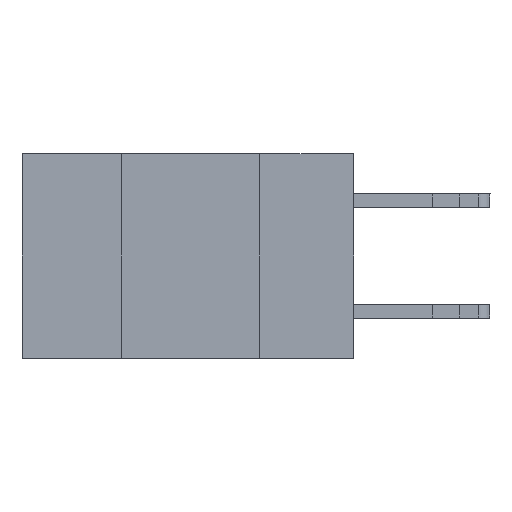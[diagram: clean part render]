
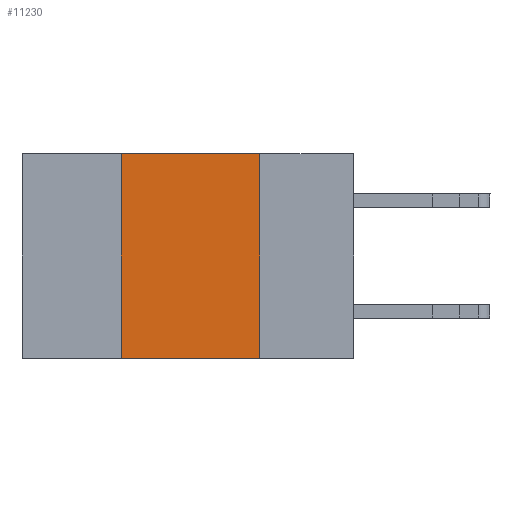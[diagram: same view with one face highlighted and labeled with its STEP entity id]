
A CAD part, left-side view. The second image highlights one B-rep face of the part: STEP entity #11230.
In plain terms, the highlighted planar face has unit normal (-1, 0, 0).
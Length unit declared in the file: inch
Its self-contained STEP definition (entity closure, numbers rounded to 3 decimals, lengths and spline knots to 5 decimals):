
#27 = VECTOR ( 'NONE', #18853, 39.37008 ) ;
#811 = VERTEX_POINT ( 'NONE', #19959 ) ;
#1040 = DIRECTION ( 'NONE',  ( 0., 0., 1. ) ) ;
#1894 = ORIENTED_EDGE ( 'NONE', *, *, #13510, .T. ) ;
#2564 = EDGE_LOOP ( 'NONE', ( #18502, #21080, #18446, #1894 ) ) ;
#2860 = DIRECTION ( 'NONE',  ( 0., -1., 0. ) ) ;
#4408 = LINE ( 'NONE', #16686, #27 ) ;
#8374 = DIRECTION ( 'NONE',  ( 1., 0., 0. ) ) ;
#9602 = AXIS2_PLACEMENT_3D ( 'NONE', #18667, #8374, #18539 ) ;
#10160 = VERTEX_POINT ( 'NONE', #21733 ) ;
#11166 = CARTESIAN_POINT ( 'NONE',  ( 0., 0.42, -0.37 ) ) ;
#11230 = ADVANCED_FACE ( 'NONE', ( #16837 ), #21931, .F. ) ;
#11403 = CARTESIAN_POINT ( 'NONE',  ( 0., 0.6, 0. ) ) ;
#11689 = EDGE_CURVE ( 'NONE', #811, #10160, #14798, .T. ) ;
#12183 = VERTEX_POINT ( 'NONE', #16342 ) ;
#13083 = DIRECTION ( 'NONE',  ( 0., -1., 0. ) ) ;
#13177 = VECTOR ( 'NONE', #1040, 39.37008 ) ;
#13510 = EDGE_CURVE ( 'NONE', #22340, #12183, #16766, .T. ) ;
#14726 = VECTOR ( 'NONE', #2860, 39.37008 ) ;
#14798 = LINE ( 'NONE', #11403, #14726 ) ;
#14912 = VECTOR ( 'NONE', #13083, 39.37008 ) ;
#16342 = CARTESIAN_POINT ( 'NONE',  ( 0., 0.17, -0.37 ) ) ;
#16686 = CARTESIAN_POINT ( 'NONE',  ( 0., 0.17, 0. ) ) ;
#16766 = LINE ( 'NONE', #22200, #14912 ) ;
#16802 = CARTESIAN_POINT ( 'NONE',  ( 0., 0.42, 0. ) ) ;
#16837 = FACE_OUTER_BOUND ( 'NONE', #2564, .T. ) ;
#18446 = ORIENTED_EDGE ( 'NONE', *, *, #20998, .F. ) ;
#18502 = ORIENTED_EDGE ( 'NONE', *, *, #19882, .F. ) ;
#18539 = DIRECTION ( 'NONE',  ( 0., 0., -1. ) ) ;
#18667 = CARTESIAN_POINT ( 'NONE',  ( 0., 0.6, 0. ) ) ;
#18853 = DIRECTION ( 'NONE',  ( 0., 0., -1. ) ) ;
#19882 = EDGE_CURVE ( 'NONE', #10160, #12183, #4408, .T. ) ;
#19959 = CARTESIAN_POINT ( 'NONE',  ( 0., 0.42, 0. ) ) ;
#20998 = EDGE_CURVE ( 'NONE', #22340, #811, #22119, .T. ) ;
#21080 = ORIENTED_EDGE ( 'NONE', *, *, #11689, .F. ) ;
#21733 = CARTESIAN_POINT ( 'NONE',  ( 0., 0.17, 0. ) ) ;
#21931 = PLANE ( 'NONE',  #9602 ) ;
#22119 = LINE ( 'NONE', #16802, #13177 ) ;
#22200 = CARTESIAN_POINT ( 'NONE',  ( 0., 0.6, -0.37 ) ) ;
#22340 = VERTEX_POINT ( 'NONE', #11166 ) ;
